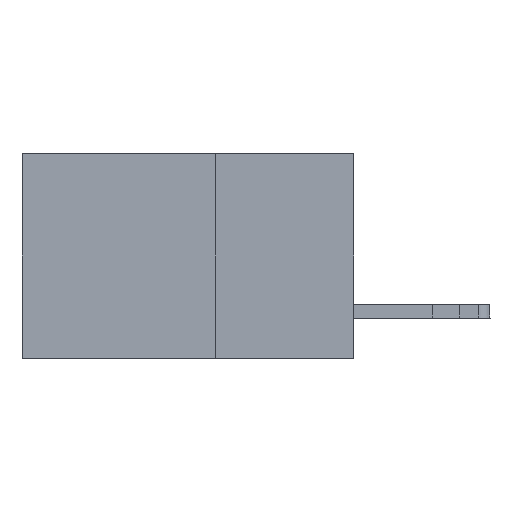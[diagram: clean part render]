
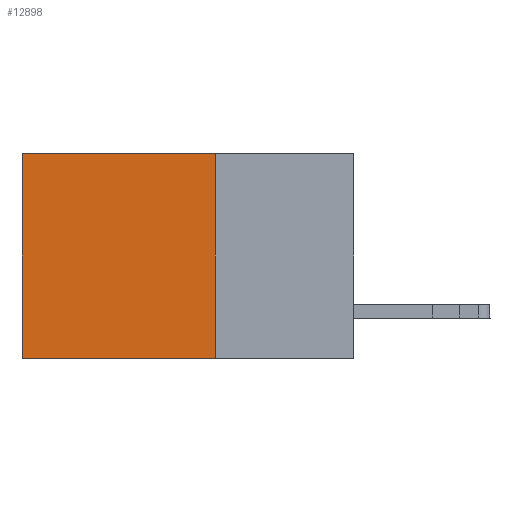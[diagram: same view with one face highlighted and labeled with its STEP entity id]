
A CAD part, left-side view. The second image highlights one B-rep face of the part: STEP entity #12898.
In plain terms, the highlighted planar face has unit normal (-1, 0, 0).
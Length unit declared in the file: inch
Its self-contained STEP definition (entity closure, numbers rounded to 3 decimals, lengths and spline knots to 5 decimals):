
#236 = EDGE_CURVE ( 'NONE', #1994, #1925, #25313, .T. ) ;
#1925 = VERTEX_POINT ( 'NONE', #26503 ) ;
#1994 = VERTEX_POINT ( 'NONE', #29345 ) ;
#2487 = VECTOR ( 'NONE', #31231, 39.37008 ) ;
#2697 = ORIENTED_EDGE ( 'NONE', *, *, #3046, .F. ) ;
#2801 = DIRECTION ( 'NONE',  ( 0., 1., 0. ) ) ;
#3046 = EDGE_CURVE ( 'NONE', #1925, #11963, #6499, .T. ) ;
#5547 = CARTESIAN_POINT ( 'NONE',  ( 0.2875, 0.6, 0. ) ) ;
#6499 = LINE ( 'NONE', #23062, #20467 ) ;
#7771 = DIRECTION ( 'NONE',  ( 0., 0., -1. ) ) ;
#8215 = VECTOR ( 'NONE', #2801, 39.37008 ) ;
#9614 = EDGE_CURVE ( 'NONE', #1994, #29276, #23007, .T. ) ;
#10341 = CARTESIAN_POINT ( 'NONE',  ( 0.2875, 0.6, 0. ) ) ;
#10592 = VECTOR ( 'NONE', #29048, 39.37008 ) ;
#11108 = AXIS2_PLACEMENT_3D ( 'NONE', #33850, #23512, #7771 ) ;
#11963 = VERTEX_POINT ( 'NONE', #23125 ) ;
#11993 = FACE_OUTER_BOUND ( 'NONE', #22125, .T. ) ;
#12898 = ADVANCED_FACE ( 'NONE', ( #11993 ), #31209, .F. ) ;
#15087 = ORIENTED_EDGE ( 'NONE', *, *, #9614, .T. ) ;
#15297 = ORIENTED_EDGE ( 'NONE', *, *, #22614, .T. ) ;
#18550 = CARTESIAN_POINT ( 'NONE',  ( 0.2875, 0.25, 0. ) ) ;
#20467 = VECTOR ( 'NONE', #33393, 39.37008 ) ;
#21338 = CARTESIAN_POINT ( 'NONE',  ( 0.2875, 0.25, 0. ) ) ;
#22125 = EDGE_LOOP ( 'NONE', ( #15297, #2697, #24293, #15087 ) ) ;
#22614 = EDGE_CURVE ( 'NONE', #29276, #11963, #30335, .T. ) ;
#23007 = LINE ( 'NONE', #18550, #8215 ) ;
#23062 = CARTESIAN_POINT ( 'NONE',  ( 0.2875, 0.25, -0.37 ) ) ;
#23125 = CARTESIAN_POINT ( 'NONE',  ( 0.2875, 0.6, -0.37 ) ) ;
#23512 = DIRECTION ( 'NONE',  ( 1., 0., 0. ) ) ;
#24293 = ORIENTED_EDGE ( 'NONE', *, *, #236, .F. ) ;
#25313 = LINE ( 'NONE', #21338, #10592 ) ;
#26503 = CARTESIAN_POINT ( 'NONE',  ( 0.2875, 0.25, -0.37 ) ) ;
#29048 = DIRECTION ( 'NONE',  ( 0., 0., -1. ) ) ;
#29276 = VERTEX_POINT ( 'NONE', #5547 ) ;
#29345 = CARTESIAN_POINT ( 'NONE',  ( 0.2875, 0.25, 0. ) ) ;
#30335 = LINE ( 'NONE', #10341, #2487 ) ;
#31209 = PLANE ( 'NONE',  #11108 ) ;
#31231 = DIRECTION ( 'NONE',  ( 0., 0., -1. ) ) ;
#33393 = DIRECTION ( 'NONE',  ( 0., 1., 0. ) ) ;
#33850 = CARTESIAN_POINT ( 'NONE',  ( 0.2875, 0.25, 0. ) ) ;
